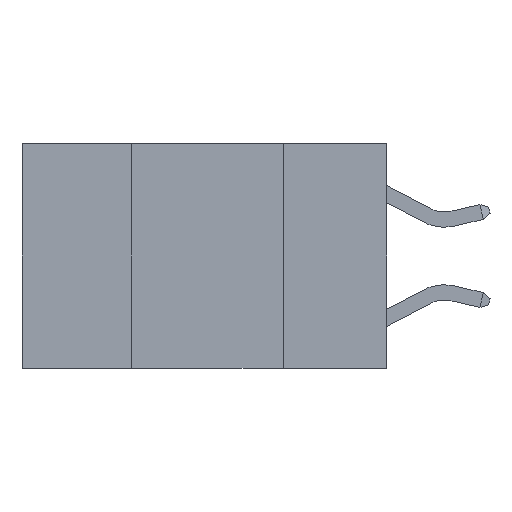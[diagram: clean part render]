
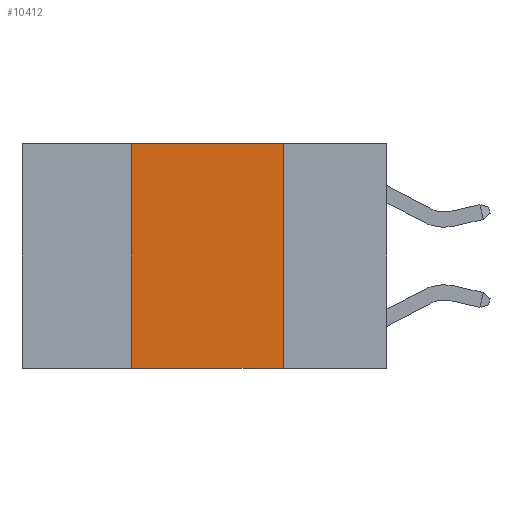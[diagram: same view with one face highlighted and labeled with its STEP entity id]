
A CAD part, left-side view. The second image highlights one B-rep face of the part: STEP entity #10412.
In plain terms, the highlighted planar face has unit normal (-1, 0, 0).
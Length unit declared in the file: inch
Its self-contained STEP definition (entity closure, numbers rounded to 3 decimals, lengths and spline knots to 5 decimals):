
#31 = LINE ( 'NONE', #8970, #5881 ) ;
#412 = PLANE ( 'NONE',  #7301 ) ;
#798 = ORIENTED_EDGE ( 'NONE', *, *, #1782, .F. ) ;
#1387 = CARTESIAN_POINT ( 'NONE',  ( 0., 0.42, -0.37 ) ) ;
#1527 = VECTOR ( 'NONE', #10985, 39.37008 ) ;
#1782 = EDGE_CURVE ( 'NONE', #5130, #13032, #31, .T. ) ;
#2031 = LINE ( 'NONE', #5227, #1527 ) ;
#2273 = DIRECTION ( 'NONE',  ( 0., -1., 0. ) ) ;
#2369 = VECTOR ( 'NONE', #8340, 39.37008 ) ;
#2546 = DIRECTION ( 'NONE',  ( 0., 0., -1. ) ) ;
#2946 = EDGE_CURVE ( 'NONE', #6176, #11172, #13620, .T. ) ;
#3460 = EDGE_CURVE ( 'NONE', #13032, #11172, #3854, .T. ) ;
#3854 = LINE ( 'NONE', #12668, #2369 ) ;
#5130 = VERTEX_POINT ( 'NONE', #7402 ) ;
#5227 = CARTESIAN_POINT ( 'NONE',  ( 0., 0.42, 0. ) ) ;
#5881 = VECTOR ( 'NONE', #13302, 39.37008 ) ;
#6176 = VERTEX_POINT ( 'NONE', #1387 ) ;
#7038 = FACE_OUTER_BOUND ( 'NONE', #10443, .T. ) ;
#7301 = AXIS2_PLACEMENT_3D ( 'NONE', #8920, #11145, #2546 ) ;
#7402 = CARTESIAN_POINT ( 'NONE',  ( 0., 0.42, 0. ) ) ;
#7794 = CARTESIAN_POINT ( 'NONE',  ( 0., 0.6, -0.37 ) ) ;
#8340 = DIRECTION ( 'NONE',  ( 0., 0., -1. ) ) ;
#8739 = CARTESIAN_POINT ( 'NONE',  ( 0., 0.17, -0.37 ) ) ;
#8920 = CARTESIAN_POINT ( 'NONE',  ( 0., 0.6, 0. ) ) ;
#8970 = CARTESIAN_POINT ( 'NONE',  ( 0., 0.6, 0. ) ) ;
#9918 = VECTOR ( 'NONE', #2273, 39.37008 ) ;
#10412 = ADVANCED_FACE ( 'NONE', ( #7038 ), #412, .F. ) ;
#10443 = EDGE_LOOP ( 'NONE', ( #12697, #798, #10446, #13171 ) ) ;
#10446 = ORIENTED_EDGE ( 'NONE', *, *, #12457, .F. ) ;
#10985 = DIRECTION ( 'NONE',  ( 0., 0., 1. ) ) ;
#11145 = DIRECTION ( 'NONE',  ( 1., 0., 0. ) ) ;
#11172 = VERTEX_POINT ( 'NONE', #8739 ) ;
#12457 = EDGE_CURVE ( 'NONE', #6176, #5130, #2031, .T. ) ;
#12668 = CARTESIAN_POINT ( 'NONE',  ( 0., 0.17, 0. ) ) ;
#12697 = ORIENTED_EDGE ( 'NONE', *, *, #3460, .F. ) ;
#13032 = VERTEX_POINT ( 'NONE', #13358 ) ;
#13171 = ORIENTED_EDGE ( 'NONE', *, *, #2946, .T. ) ;
#13302 = DIRECTION ( 'NONE',  ( 0., -1., 0. ) ) ;
#13358 = CARTESIAN_POINT ( 'NONE',  ( 0., 0.17, 0. ) ) ;
#13620 = LINE ( 'NONE', #7794, #9918 ) ;
